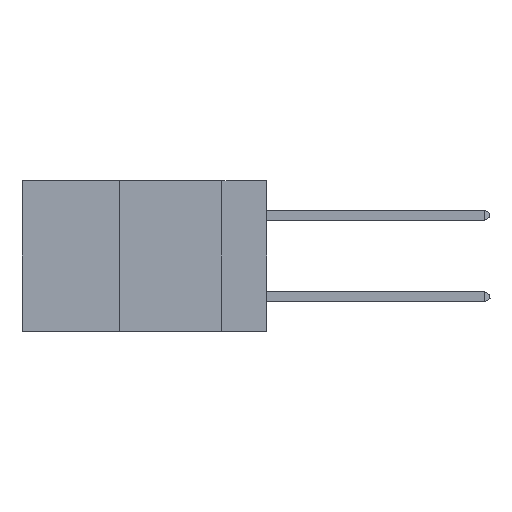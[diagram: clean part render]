
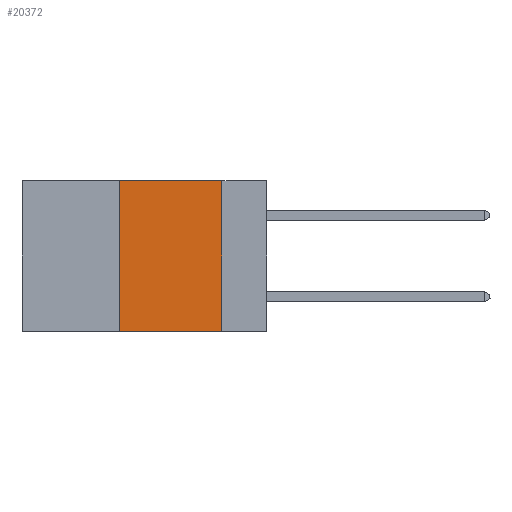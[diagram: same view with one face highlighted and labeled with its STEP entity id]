
A CAD part, left-side view. The second image highlights one B-rep face of the part: STEP entity #20372.
In plain terms, the highlighted planar face has unit normal (-1, 0, 0).
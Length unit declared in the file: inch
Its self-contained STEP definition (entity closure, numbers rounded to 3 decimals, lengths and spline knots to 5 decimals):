
#4276 = DIRECTION ( 'NONE',  ( 0., 0., -1. ) ) ;
#7328 = EDGE_LOOP ( 'NONE', ( #27163, #21416, #36331, #20519 ) ) ;
#7611 = AXIS2_PLACEMENT_3D ( 'NONE', #28143, #16204, #10393 ) ;
#8080 = VERTEX_POINT ( 'NONE', #22490 ) ;
#8290 = CARTESIAN_POINT ( 'NONE',  ( 0., 0.11, -0.37 ) ) ;
#8539 = CARTESIAN_POINT ( 'NONE',  ( 0., 0.36, 0. ) ) ;
#9052 = EDGE_CURVE ( 'NONE', #32565, #22331, #21446, .T. ) ;
#9388 = PLANE ( 'NONE',  #7611 ) ;
#10393 = DIRECTION ( 'NONE',  ( 0., 0., -1. ) ) ;
#12628 = DIRECTION ( 'NONE',  ( 0., -1., 0. ) ) ;
#14765 = CARTESIAN_POINT ( 'NONE',  ( 0., 0.6, 0. ) ) ;
#16170 = VERTEX_POINT ( 'NONE', #8290 ) ;
#16204 = DIRECTION ( 'NONE',  ( 1., 0., 0. ) ) ;
#16455 = VECTOR ( 'NONE', #28548, 39.37008 ) ;
#17277 = VECTOR ( 'NONE', #12628, 39.37008 ) ;
#18582 = EDGE_CURVE ( 'NONE', #22331, #16170, #29392, .T. ) ;
#18650 = CARTESIAN_POINT ( 'NONE',  ( 0., 0.36, 0. ) ) ;
#20372 = ADVANCED_FACE ( 'NONE', ( #22792 ), #9388, .F. ) ;
#20519 = ORIENTED_EDGE ( 'NONE', *, *, #35345, .T. ) ;
#21015 = LINE ( 'NONE', #18650, #22458 ) ;
#21416 = ORIENTED_EDGE ( 'NONE', *, *, #9052, .F. ) ;
#21446 = LINE ( 'NONE', #14765, #17277 ) ;
#21561 = LINE ( 'NONE', #22452, #16455 ) ;
#21981 = CARTESIAN_POINT ( 'NONE',  ( 0., 0.11, 0. ) ) ;
#22331 = VERTEX_POINT ( 'NONE', #30274 ) ;
#22452 = CARTESIAN_POINT ( 'NONE',  ( 0., 0.6, -0.37 ) ) ;
#22458 = VECTOR ( 'NONE', #24873, 39.37008 ) ;
#22490 = CARTESIAN_POINT ( 'NONE',  ( 0., 0.36, -0.37 ) ) ;
#22792 = FACE_OUTER_BOUND ( 'NONE', #7328, .T. ) ;
#24873 = DIRECTION ( 'NONE',  ( 0., 0., 1. ) ) ;
#27163 = ORIENTED_EDGE ( 'NONE', *, *, #18582, .F. ) ;
#28143 = CARTESIAN_POINT ( 'NONE',  ( 0., 0.6, 0. ) ) ;
#28548 = DIRECTION ( 'NONE',  ( 0., -1., 0. ) ) ;
#29392 = LINE ( 'NONE', #21981, #32174 ) ;
#30274 = CARTESIAN_POINT ( 'NONE',  ( 0., 0.11, 0. ) ) ;
#32174 = VECTOR ( 'NONE', #4276, 39.37008 ) ;
#32565 = VERTEX_POINT ( 'NONE', #8539 ) ;
#35345 = EDGE_CURVE ( 'NONE', #8080, #16170, #21561, .T. ) ;
#35907 = EDGE_CURVE ( 'NONE', #8080, #32565, #21015, .T. ) ;
#36331 = ORIENTED_EDGE ( 'NONE', *, *, #35907, .F. ) ;
